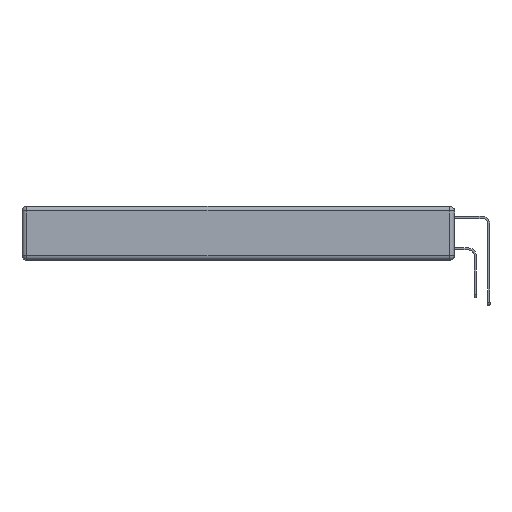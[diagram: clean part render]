
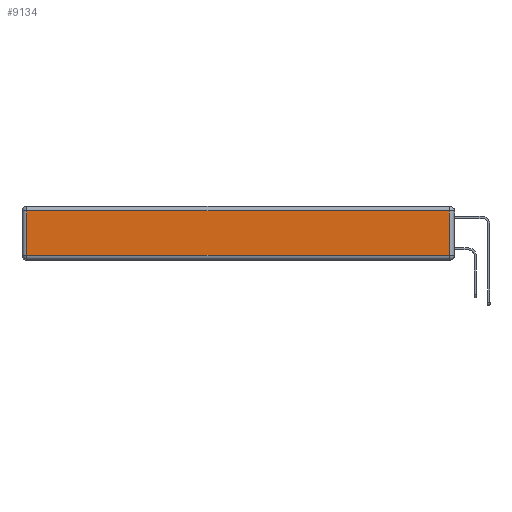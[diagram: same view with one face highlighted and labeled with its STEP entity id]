
A CAD part, left-side view. The second image highlights one B-rep face of the part: STEP entity #9134.
In plain terms, the highlighted planar face has unit normal (-1, 0, 0).
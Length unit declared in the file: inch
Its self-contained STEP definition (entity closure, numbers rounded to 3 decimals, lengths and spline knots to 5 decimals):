
#54 = ORIENTED_EDGE ( 'NONE', *, *, #1190, .T. ) ;
#533 = ORIENTED_EDGE ( 'NONE', *, *, #8183, .T. ) ;
#916 = VECTOR ( 'NONE', #2258, 39.37008 ) ;
#1190 = EDGE_CURVE ( 'NONE', #15275, #11742, #11705, .T. ) ;
#1899 = CARTESIAN_POINT ( 'NONE',  ( 0., 0.03, -0.343 ) ) ;
#2258 = DIRECTION ( 'NONE',  ( 0., 0., -1. ) ) ;
#2310 = CARTESIAN_POINT ( 'NONE',  ( 0., 0., -0.313 ) ) ;
#2653 = EDGE_LOOP ( 'NONE', ( #10163, #7235, #533, #54 ) ) ;
#3153 = EDGE_CURVE ( 'NONE', #12715, #11329, #8191, .T. ) ;
#3487 = FACE_OUTER_BOUND ( 'NONE', #2653, .T. ) ;
#4235 = CARTESIAN_POINT ( 'NONE',  ( 0., 2.72, -0.03 ) ) ;
#4671 = CARTESIAN_POINT ( 'NONE',  ( 0., 0., -0.343 ) ) ;
#4672 = DIRECTION ( 'NONE',  ( 0., -1., 0. ) ) ;
#5422 = DIRECTION ( 'NONE',  ( 0., 1., 0. ) ) ;
#5861 = DIRECTION ( 'NONE',  ( -1., 0., 0. ) ) ;
#7235 = ORIENTED_EDGE ( 'NONE', *, *, #3153, .T. ) ;
#7343 = PLANE ( 'NONE',  #12767 ) ;
#7346 = LINE ( 'NONE', #2310, #10536 ) ;
#7795 = LINE ( 'NONE', #12593, #10125 ) ;
#7920 = CARTESIAN_POINT ( 'NONE',  ( 0., 0.03, -0.03 ) ) ;
#8183 = EDGE_CURVE ( 'NONE', #11329, #15275, #7795, .T. ) ;
#8191 = LINE ( 'NONE', #1899, #11435 ) ;
#9134 = ADVANCED_FACE ( 'NONE', ( #3487 ), #7343, .T. ) ;
#9784 = DIRECTION ( 'NONE',  ( 0., 0., 1. ) ) ;
#10014 = CARTESIAN_POINT ( 'NONE',  ( 0., 2.72, -0.313 ) ) ;
#10125 = VECTOR ( 'NONE', #5422, 39.37008 ) ;
#10163 = ORIENTED_EDGE ( 'NONE', *, *, #11469, .T. ) ;
#10536 = VECTOR ( 'NONE', #4672, 39.37008 ) ;
#11329 = VERTEX_POINT ( 'NONE', #7920 ) ;
#11435 = VECTOR ( 'NONE', #12747, 39.37008 ) ;
#11469 = EDGE_CURVE ( 'NONE', #11742, #12715, #7346, .T. ) ;
#11693 = CARTESIAN_POINT ( 'NONE',  ( 0., 0.03, -0.313 ) ) ;
#11705 = LINE ( 'NONE', #13047, #916 ) ;
#11742 = VERTEX_POINT ( 'NONE', #10014 ) ;
#12593 = CARTESIAN_POINT ( 'NONE',  ( 0., 2.75, -0.03 ) ) ;
#12715 = VERTEX_POINT ( 'NONE', #11693 ) ;
#12747 = DIRECTION ( 'NONE',  ( 0., 0., 1. ) ) ;
#12767 = AXIS2_PLACEMENT_3D ( 'NONE', #4671, #5861, #9784 ) ;
#13047 = CARTESIAN_POINT ( 'NONE',  ( 0., 2.72, -0.343 ) ) ;
#15275 = VERTEX_POINT ( 'NONE', #4235 ) ;
